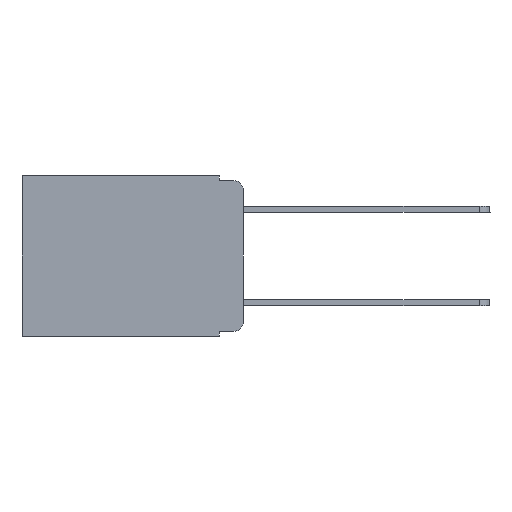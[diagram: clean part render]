
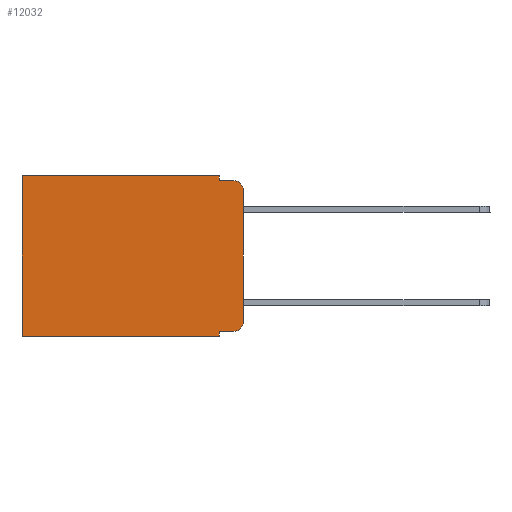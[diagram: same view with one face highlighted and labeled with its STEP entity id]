
A CAD part, left-side view. The second image highlights one B-rep face of the part: STEP entity #12032.
In plain terms, the highlighted planar face has unit normal (-1, 0, 0).
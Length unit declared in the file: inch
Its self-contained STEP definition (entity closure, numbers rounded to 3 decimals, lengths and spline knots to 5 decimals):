
#605 = DIRECTION ( 'NONE',  ( 0., 0., -1. ) ) ;
#666 = CARTESIAN_POINT ( 'NONE',  ( 0.298, 0.473, 0. ) ) ;
#1042 = VECTOR ( 'NONE', #15718, 39.37008 ) ;
#1166 = ORIENTED_EDGE ( 'NONE', *, *, #13580, .F. ) ;
#1318 = CARTESIAN_POINT ( 'NONE',  ( 0.298, 0.02, -0.01 ) ) ;
#1351 = VECTOR ( 'NONE', #4020, 39.37008 ) ;
#1648 = VERTEX_POINT ( 'NONE', #1318 ) ;
#1664 = CIRCLE ( 'NONE', #14102, 0.02 ) ;
#1734 = DIRECTION ( 'NONE',  ( 0., 0., -1. ) ) ;
#1802 = DIRECTION ( 'NONE',  ( 0., 0., -1. ) ) ;
#1875 = CARTESIAN_POINT ( 'NONE',  ( 0.298, 0.02, -0.03 ) ) ;
#2490 = ORIENTED_EDGE ( 'NONE', *, *, #9189, .T. ) ;
#2787 = AXIS2_PLACEMENT_3D ( 'NONE', #1875, #14097, #4403 ) ;
#2792 = CARTESIAN_POINT ( 'NONE',  ( 0.298, 0.051, 0. ) ) ;
#2936 = CARTESIAN_POINT ( 'NONE',  ( 0.298, 0.051, -0.333 ) ) ;
#3266 = VERTEX_POINT ( 'NONE', #15801 ) ;
#3380 = CARTESIAN_POINT ( 'NONE',  ( 0.298, 0.051, 0. ) ) ;
#3709 = EDGE_CURVE ( 'NONE', #9016, #14172, #13239, .T. ) ;
#4020 = DIRECTION ( 'NONE',  ( 0., 1., 0. ) ) ;
#4194 = EDGE_CURVE ( 'NONE', #16359, #11987, #4893, .T. ) ;
#4274 = CARTESIAN_POINT ( 'NONE',  ( 0.298, 0., -0.313 ) ) ;
#4403 = DIRECTION ( 'NONE',  ( 0., 0., -1. ) ) ;
#4431 = EDGE_CURVE ( 'NONE', #8851, #1648, #15625, .T. ) ;
#4497 = VECTOR ( 'NONE', #11605, 39.37008 ) ;
#4527 = DIRECTION ( 'NONE',  ( 0., -1., 0. ) ) ;
#4830 = DIRECTION ( 'NONE',  ( 0., 0., -1. ) ) ;
#4893 = LINE ( 'NONE', #6078, #4497 ) ;
#5045 = EDGE_CURVE ( 'NONE', #15365, #9016, #14601, .T. ) ;
#5134 = EDGE_LOOP ( 'NONE', ( #15035, #13808, #17477, #5293, #13203, #5923, #1166, #14292, #2490, #10828 ) ) ;
#5293 = ORIENTED_EDGE ( 'NONE', *, *, #7381, .F. ) ;
#5923 = ORIENTED_EDGE ( 'NONE', *, *, #3709, .T. ) ;
#6078 = CARTESIAN_POINT ( 'NONE',  ( 0.298, 0.051, 0. ) ) ;
#6197 = DIRECTION ( 'NONE',  ( 0., 0., -1. ) ) ;
#6610 = AXIS2_PLACEMENT_3D ( 'NONE', #8929, #10208, #605 ) ;
#6747 = CARTESIAN_POINT ( 'NONE',  ( 0.298, 0., -0.343 ) ) ;
#7268 = CARTESIAN_POINT ( 'NONE',  ( 0.298, 0.473, -0.343 ) ) ;
#7381 = EDGE_CURVE ( 'NONE', #15365, #8851, #10268, .T. ) ;
#7750 = CARTESIAN_POINT ( 'NONE',  ( 0.298, 0.051, -0.343 ) ) ;
#8181 = CARTESIAN_POINT ( 'NONE',  ( 0.298, 0.473, 0. ) ) ;
#8192 = CARTESIAN_POINT ( 'NONE',  ( 0.298, 0., -0.03 ) ) ;
#8851 = VERTEX_POINT ( 'NONE', #17179 ) ;
#8881 = CARTESIAN_POINT ( 'NONE',  ( 0.298, 0.02, -0.313 ) ) ;
#8929 = CARTESIAN_POINT ( 'NONE',  ( 0.298, 0., 0. ) ) ;
#9016 = VERTEX_POINT ( 'NONE', #8181 ) ;
#9183 = FACE_OUTER_BOUND ( 'NONE', #5134, .T. ) ;
#9189 = EDGE_CURVE ( 'NONE', #16359, #3266, #10155, .T. ) ;
#10126 = LINE ( 'NONE', #17289, #12650 ) ;
#10155 = LINE ( 'NONE', #11426, #14657 ) ;
#10208 = DIRECTION ( 'NONE',  ( 1., 0., 0. ) ) ;
#10221 = VECTOR ( 'NONE', #4830, 39.37008 ) ;
#10268 = LINE ( 'NONE', #3380, #16884 ) ;
#10828 = ORIENTED_EDGE ( 'NONE', *, *, #10942, .T. ) ;
#10942 = EDGE_CURVE ( 'NONE', #3266, #14579, #1664, .T. ) ;
#11426 = CARTESIAN_POINT ( 'NONE',  ( 0.298, 0.051, -0.333 ) ) ;
#11464 = CARTESIAN_POINT ( 'NONE',  ( 0.298, 0.051, -0.01 ) ) ;
#11605 = DIRECTION ( 'NONE',  ( 0., 0., -1. ) ) ;
#11634 = DIRECTION ( 'NONE',  ( 0., 1., 0. ) ) ;
#11986 = VECTOR ( 'NONE', #11634, 39.37008 ) ;
#11987 = VERTEX_POINT ( 'NONE', #7750 ) ;
#12032 = ADVANCED_FACE ( 'NONE', ( #9183 ), #14372, .F. ) ;
#12650 = VECTOR ( 'NONE', #1802, 39.37008 ) ;
#12783 = DIRECTION ( 'NONE',  ( -1., 0., 0. ) ) ;
#12919 = CIRCLE ( 'NONE', #2787, 0.02 ) ;
#13159 = CARTESIAN_POINT ( 'NONE',  ( 0.298, 0., 0. ) ) ;
#13203 = ORIENTED_EDGE ( 'NONE', *, *, #5045, .T. ) ;
#13239 = LINE ( 'NONE', #666, #10221 ) ;
#13277 = EDGE_CURVE ( 'NONE', #13555, #1648, #12919, .T. ) ;
#13555 = VERTEX_POINT ( 'NONE', #8192 ) ;
#13580 = EDGE_CURVE ( 'NONE', #11987, #14172, #17892, .T. ) ;
#13808 = ORIENTED_EDGE ( 'NONE', *, *, #13277, .T. ) ;
#14097 = DIRECTION ( 'NONE',  ( -1., 0., 0. ) ) ;
#14102 = AXIS2_PLACEMENT_3D ( 'NONE', #8881, #12783, #1734 ) ;
#14172 = VERTEX_POINT ( 'NONE', #7268 ) ;
#14278 = EDGE_CURVE ( 'NONE', #13555, #14579, #10126, .T. ) ;
#14292 = ORIENTED_EDGE ( 'NONE', *, *, #4194, .F. ) ;
#14372 = PLANE ( 'NONE',  #6610 ) ;
#14579 = VERTEX_POINT ( 'NONE', #4274 ) ;
#14601 = LINE ( 'NONE', #13159, #11986 ) ;
#14657 = VECTOR ( 'NONE', #4527, 39.37008 ) ;
#15035 = ORIENTED_EDGE ( 'NONE', *, *, #14278, .F. ) ;
#15365 = VERTEX_POINT ( 'NONE', #2792 ) ;
#15625 = LINE ( 'NONE', #11464, #1042 ) ;
#15718 = DIRECTION ( 'NONE',  ( 0., -1., 0. ) ) ;
#15801 = CARTESIAN_POINT ( 'NONE',  ( 0.298, 0.02, -0.333 ) ) ;
#16359 = VERTEX_POINT ( 'NONE', #2936 ) ;
#16884 = VECTOR ( 'NONE', #6197, 39.37008 ) ;
#17179 = CARTESIAN_POINT ( 'NONE',  ( 0.298, 0.051, -0.01 ) ) ;
#17289 = CARTESIAN_POINT ( 'NONE',  ( 0.298, 0., 0. ) ) ;
#17477 = ORIENTED_EDGE ( 'NONE', *, *, #4431, .F. ) ;
#17892 = LINE ( 'NONE', #6747, #1351 ) ;
